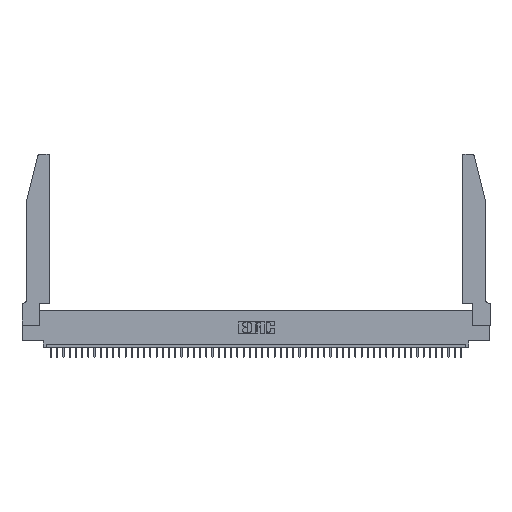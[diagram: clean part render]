
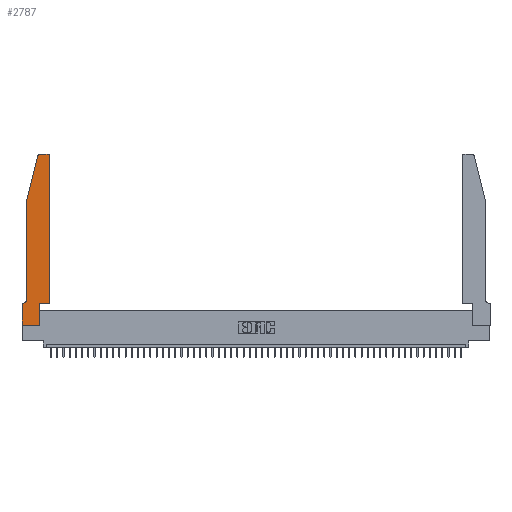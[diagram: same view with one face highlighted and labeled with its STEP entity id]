
A CAD part, top view. The second image highlights one B-rep face of the part: STEP entity #2787.
In plain terms, the highlighted planar face has unit normal (0, 0, 1).
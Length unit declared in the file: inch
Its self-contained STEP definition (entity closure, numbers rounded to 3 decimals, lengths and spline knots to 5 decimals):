
#55 = VECTOR ( 'NONE', #39803, 39.37008 ) ;
#1900 = FACE_OUTER_BOUND ( 'NONE', #35424, .T. ) ;
#2498 = PLANE ( 'NONE',  #36843 ) ;
#2787 = ADVANCED_FACE ( 'NONE', ( #1900 ), #2498, .T. ) ;
#2905 = ORIENTED_EDGE ( 'NONE', *, *, #9594, .T. ) ;
#4176 = EDGE_CURVE ( 'NONE', #50229, #10527, #47741, .T. ) ;
#5252 = VECTOR ( 'NONE', #48611, 39.37008 ) ;
#5687 = LINE ( 'NONE', #28325, #10775 ) ;
#6175 = CARTESIAN_POINT ( 'NONE',  ( 0.4205, 2.72, 0.37 ) ) ;
#7583 = DIRECTION ( 'NONE',  ( 0., 0., 1. ) ) ;
#7810 = CARTESIAN_POINT ( 'NONE',  ( 0.4505, 0.35, 0.37 ) ) ;
#8803 = CIRCLE ( 'NONE', #41083, 0.03 ) ;
#8973 = CARTESIAN_POINT ( 'NONE',  ( 0.25487, 2.72718, 0.37 ) ) ;
#9594 = EDGE_CURVE ( 'NONE', #10527, #15590, #43870, .T. ) ;
#9976 = EDGE_CURVE ( 'NONE', #10679, #14499, #11161, .T. ) ;
#10025 = DIRECTION ( 'NONE',  ( 1., 0., 0. ) ) ;
#10091 = DIRECTION ( 'NONE',  ( 0., 1., 0. ) ) ;
#10218 = CARTESIAN_POINT ( 'NONE',  ( 0., 0., 0.37 ) ) ;
#10527 = VERTEX_POINT ( 'NONE', #15953 ) ;
#10679 = VERTEX_POINT ( 'NONE', #8973 ) ;
#10714 = LINE ( 'NONE', #38359, #55 ) ;
#10775 = VECTOR ( 'NONE', #10091, 39.37008 ) ;
#11161 = LINE ( 'NONE', #41661, #31827 ) ;
#11325 = DIRECTION ( 'NONE',  ( -1., 0., 0. ) ) ;
#12200 = CARTESIAN_POINT ( 'NONE',  ( 0.4205, 2.75, 0.37 ) ) ;
#12210 = ORIENTED_EDGE ( 'NONE', *, *, #13609, .T. ) ;
#12827 = CARTESIAN_POINT ( 'NONE',  ( 0., 0., 0.37 ) ) ;
#13609 = EDGE_CURVE ( 'NONE', #14499, #44022, #10714, .T. ) ;
#14098 = LINE ( 'NONE', #30967, #23520 ) ;
#14166 = LINE ( 'NONE', #36131, #5252 ) ;
#14499 = VERTEX_POINT ( 'NONE', #33641 ) ;
#14751 = CARTESIAN_POINT ( 'NONE',  ( 0.0755, 0.42, 0.37 ) ) ;
#15590 = VERTEX_POINT ( 'NONE', #12200 ) ;
#15953 = CARTESIAN_POINT ( 'NONE',  ( 0.4505, 2.72, 0.37 ) ) ;
#17326 = ORIENTED_EDGE ( 'NONE', *, *, #18371, .T. ) ;
#17549 = ORIENTED_EDGE ( 'NONE', *, *, #28271, .T. ) ;
#17560 = CARTESIAN_POINT ( 'NONE',  ( 0.4505, 0.35, 0.37 ) ) ;
#17607 = DIRECTION ( 'NONE',  ( -0.239, -0.971, 0. ) ) ;
#18371 = EDGE_CURVE ( 'NONE', #30225, #36277, #14098, .T. ) ;
#18681 = DIRECTION ( 'NONE',  ( 0., 0., 1. ) ) ;
#18842 = DIRECTION ( 'NONE',  ( 0., -1., 0. ) ) ;
#21105 = ORIENTED_EDGE ( 'NONE', *, *, #21980, .T. ) ;
#21980 = EDGE_CURVE ( 'NONE', #28435, #23475, #5687, .T. ) ;
#22032 = VECTOR ( 'NONE', #10025, 39.37008 ) ;
#22040 = EDGE_CURVE ( 'NONE', #36814, #10679, #8803, .T. ) ;
#22720 = DIRECTION ( 'NONE',  ( 1., 0., 0. ) ) ;
#23475 = VERTEX_POINT ( 'NONE', #35944 ) ;
#23520 = VECTOR ( 'NONE', #11325, 39.37008 ) ;
#23956 = ORIENTED_EDGE ( 'NONE', *, *, #25319, .T. ) ;
#25319 = EDGE_CURVE ( 'NONE', #15590, #36814, #14166, .T. ) ;
#26596 = CARTESIAN_POINT ( 'NONE',  ( 0.4505, 0.35, 0.37 ) ) ;
#27490 = VECTOR ( 'NONE', #39190, 39.37008 ) ;
#28136 = ORIENTED_EDGE ( 'NONE', *, *, #22040, .T. ) ;
#28271 = EDGE_CURVE ( 'NONE', #36277, #48957, #43998, .T. ) ;
#28325 = CARTESIAN_POINT ( 'NONE',  ( 0.2865, 0.35, 0.37 ) ) ;
#28435 = VERTEX_POINT ( 'NONE', #33696 ) ;
#29281 = LINE ( 'NONE', #32951, #27490 ) ;
#29993 = CARTESIAN_POINT ( 'NONE',  ( 0.0055, 0.42, 0.37 ) ) ;
#30225 = VERTEX_POINT ( 'NONE', #41064 ) ;
#30326 = ORIENTED_EDGE ( 'NONE', *, *, #9976, .T. ) ;
#30588 = CARTESIAN_POINT ( 'NONE',  ( 0., 0.35, 0.37 ) ) ;
#30967 = CARTESIAN_POINT ( 'NONE',  ( 0.0755, 0.35, 0.37 ) ) ;
#31061 = ORIENTED_EDGE ( 'NONE', *, *, #36481, .T. ) ;
#31827 = VECTOR ( 'NONE', #17607, 39.37008 ) ;
#32951 = CARTESIAN_POINT ( 'NONE',  ( 0., 0., 0.37 ) ) ;
#33639 = EDGE_CURVE ( 'NONE', #44022, #30225, #50436, .T. ) ;
#33641 = CARTESIAN_POINT ( 'NONE',  ( 0.0755, 2., 0.37 ) ) ;
#33696 = CARTESIAN_POINT ( 'NONE',  ( 0.2865, 0., 0.37 ) ) ;
#33926 = LINE ( 'NONE', #26596, #22032 ) ;
#34031 = CARTESIAN_POINT ( 'NONE',  ( 0., 0.35, 0.37 ) ) ;
#34260 = DIRECTION ( 'NONE',  ( 0., 0., 1. ) ) ;
#35334 = AXIS2_PLACEMENT_3D ( 'NONE', #6175, #34260, #46398 ) ;
#35424 = EDGE_LOOP ( 'NONE', ( #23956, #28136, #30326, #12210, #37686, #17326, #17549, #31061, #21105, #40815, #50831, #2905 ) ) ;
#35944 = CARTESIAN_POINT ( 'NONE',  ( 0.2865, 0.35, 0.37 ) ) ;
#36131 = CARTESIAN_POINT ( 'NONE',  ( 0.2605, 2.75, 0.37 ) ) ;
#36171 = CARTESIAN_POINT ( 'NONE',  ( 0.284, 2.72, 0.37 ) ) ;
#36277 = VERTEX_POINT ( 'NONE', #34031 ) ;
#36481 = EDGE_CURVE ( 'NONE', #48957, #28435, #29281, .T. ) ;
#36814 = VERTEX_POINT ( 'NONE', #51586 ) ;
#36843 = AXIS2_PLACEMENT_3D ( 'NONE', #30588, #18681, #22720 ) ;
#37686 = ORIENTED_EDGE ( 'NONE', *, *, #33639, .T. ) ;
#38359 = CARTESIAN_POINT ( 'NONE',  ( 0.0755, 2., 0.37 ) ) ;
#39190 = DIRECTION ( 'NONE',  ( 1., 0., 0. ) ) ;
#39803 = DIRECTION ( 'NONE',  ( 0., -1., 0. ) ) ;
#39971 = DIRECTION ( 'NONE',  ( 0., 1., 0. ) ) ;
#40815 = ORIENTED_EDGE ( 'NONE', *, *, #46612, .T. ) ;
#41064 = CARTESIAN_POINT ( 'NONE',  ( 0.0055, 0.35, 0.37 ) ) ;
#41083 = AXIS2_PLACEMENT_3D ( 'NONE', #36171, #7583, #43943 ) ;
#41661 = CARTESIAN_POINT ( 'NONE',  ( 0.0755, 2., 0.37 ) ) ;
#41795 = DIRECTION ( 'NONE',  ( -1., 0., 0. ) ) ;
#42731 = VECTOR ( 'NONE', #39971, 39.37008 ) ;
#43870 = CIRCLE ( 'NONE', #35334, 0.03 ) ;
#43943 = DIRECTION ( 'NONE',  ( 1., 0., 0. ) ) ;
#43998 = LINE ( 'NONE', #10218, #49600 ) ;
#44022 = VERTEX_POINT ( 'NONE', #14751 ) ;
#46398 = DIRECTION ( 'NONE',  ( 1., 0., 0. ) ) ;
#46612 = EDGE_CURVE ( 'NONE', #23475, #50229, #33926, .T. ) ;
#47741 = LINE ( 'NONE', #7810, #42731 ) ;
#48611 = DIRECTION ( 'NONE',  ( -1., 0., 0. ) ) ;
#48957 = VERTEX_POINT ( 'NONE', #12827 ) ;
#49136 = AXIS2_PLACEMENT_3D ( 'NONE', #29993, #49856, #41795 ) ;
#49600 = VECTOR ( 'NONE', #18842, 39.37008 ) ;
#49856 = DIRECTION ( 'NONE',  ( 0., 0., -1. ) ) ;
#50229 = VERTEX_POINT ( 'NONE', #17560 ) ;
#50436 = CIRCLE ( 'NONE', #49136, 0.07 ) ;
#50831 = ORIENTED_EDGE ( 'NONE', *, *, #4176, .T. ) ;
#51586 = CARTESIAN_POINT ( 'NONE',  ( 0.284, 2.75, 0.37 ) ) ;
